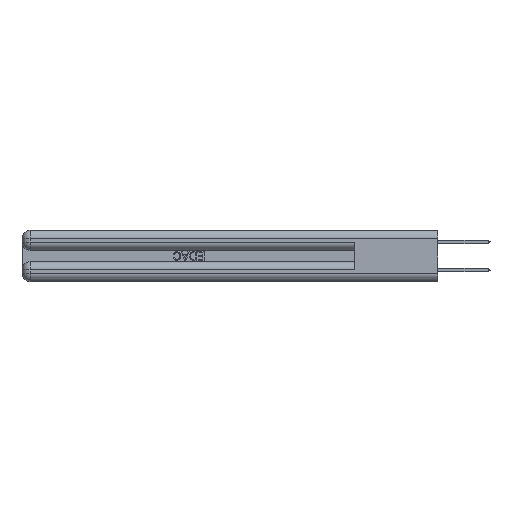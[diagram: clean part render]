
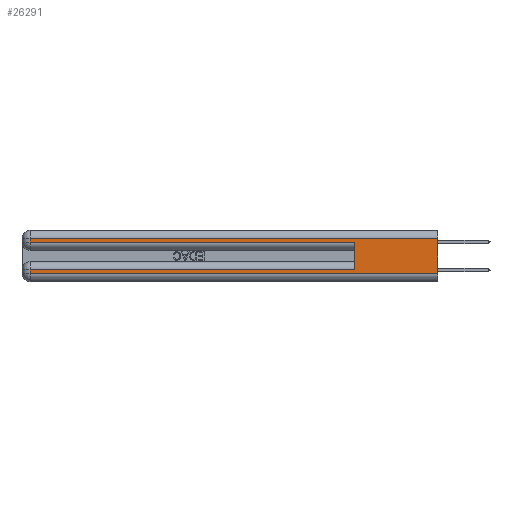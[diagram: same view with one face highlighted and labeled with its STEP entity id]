
A CAD part, left-side view. The second image highlights one B-rep face of the part: STEP entity #26291.
In plain terms, the highlighted planar face has unit normal (-1, 0, 0).
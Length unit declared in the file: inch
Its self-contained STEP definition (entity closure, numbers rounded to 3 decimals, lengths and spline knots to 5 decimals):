
#2 = LINE ( 'NONE', #25850, #28839 ) ;
#369 = VECTOR ( 'NONE', #11757, 39.37008 ) ;
#600 = CARTESIAN_POINT ( 'NONE',  ( 0., 0.6, 0.145 ) ) ;
#772 = VECTOR ( 'NONE', #30301, 39.37008 ) ;
#1163 = VERTEX_POINT ( 'NONE', #36578 ) ;
#1802 = VERTEX_POINT ( 'NONE', #23106 ) ;
#1910 = ORIENTED_EDGE ( 'NONE', *, *, #41942, .T. ) ;
#1934 = VERTEX_POINT ( 'NONE', #13478 ) ;
#3062 = CARTESIAN_POINT ( 'NONE',  ( 0., 2.94, 0.37 ) ) ;
#4387 = ORIENTED_EDGE ( 'NONE', *, *, #6411, .F. ) ;
#6411 = EDGE_CURVE ( 'NONE', #28365, #1802, #38617, .T. ) ;
#6689 = DIRECTION ( 'NONE',  ( 0., 0., -1. ) ) ;
#7509 = CARTESIAN_POINT ( 'NONE',  ( 0., 0., 0.285 ) ) ;
#8891 = CARTESIAN_POINT ( 'NONE',  ( 0., 2.94, 0.31 ) ) ;
#9011 = LINE ( 'NONE', #25058, #9567 ) ;
#9567 = VECTOR ( 'NONE', #35332, 39.37008 ) ;
#9829 = VERTEX_POINT ( 'NONE', #22189 ) ;
#9952 = EDGE_CURVE ( 'NONE', #9829, #1163, #9011, .T. ) ;
#9996 = DIRECTION ( 'NONE',  ( 0., -1., 0. ) ) ;
#11056 = CARTESIAN_POINT ( 'NONE',  ( 0., 0.6, 0.085 ) ) ;
#11757 = DIRECTION ( 'NONE',  ( 0., 0., -1. ) ) ;
#12996 = ORIENTED_EDGE ( 'NONE', *, *, #14078, .T. ) ;
#13316 = AXIS2_PLACEMENT_3D ( 'NONE', #23439, #39972, #6689 ) ;
#13478 = CARTESIAN_POINT ( 'NONE',  ( 0., 2.94, 0.285 ) ) ;
#13574 = DIRECTION ( 'NONE',  ( 0., 0., -1. ) ) ;
#13687 = VECTOR ( 'NONE', #9996, 39.37008 ) ;
#14078 = EDGE_CURVE ( 'NONE', #22019, #1163, #42571, .T. ) ;
#14930 = ORIENTED_EDGE ( 'NONE', *, *, #9952, .F. ) ;
#15753 = ORIENTED_EDGE ( 'NONE', *, *, #27311, .T. ) ;
#16132 = VECTOR ( 'NONE', #34354, 39.37008 ) ;
#17085 = EDGE_CURVE ( 'NONE', #28787, #22019, #27683, .T. ) ;
#17347 = LINE ( 'NONE', #3062, #39351 ) ;
#20038 = PLANE ( 'NONE',  #13316 ) ;
#20421 = ORIENTED_EDGE ( 'NONE', *, *, #34369, .T. ) ;
#21148 = CARTESIAN_POINT ( 'NONE',  ( 0., 2.94, 0.37 ) ) ;
#21474 = DIRECTION ( 'NONE',  ( 0., 1., 0. ) ) ;
#21560 = LINE ( 'NONE', #24256, #30461 ) ;
#22019 = VERTEX_POINT ( 'NONE', #38361 ) ;
#22189 = CARTESIAN_POINT ( 'NONE',  ( 0., 0., 0.31 ) ) ;
#22671 = CARTESIAN_POINT ( 'NONE',  ( 0., 2.94, 0.085 ) ) ;
#23106 = CARTESIAN_POINT ( 'NONE',  ( 0., 0.6, 0.285 ) ) ;
#23439 = CARTESIAN_POINT ( 'NONE',  ( 0., 0., 0.37 ) ) ;
#24256 = CARTESIAN_POINT ( 'NONE',  ( 0., 0., 0.085 ) ) ;
#25058 = CARTESIAN_POINT ( 'NONE',  ( 0., 0., 0.37 ) ) ;
#25850 = CARTESIAN_POINT ( 'NONE',  ( 0., 0., 0.31 ) ) ;
#26291 = ADVANCED_FACE ( 'NONE', ( #32659 ), #20038, .F. ) ;
#26771 = EDGE_LOOP ( 'NONE', ( #14930, #15753, #35998, #1910, #4387, #20421, #32830, #12996 ) ) ;
#27311 = EDGE_CURVE ( 'NONE', #9829, #42924, #2, .T. ) ;
#27683 = LINE ( 'NONE', #21148, #369 ) ;
#28224 = EDGE_CURVE ( 'NONE', #42924, #1934, #17347, .T. ) ;
#28365 = VERTEX_POINT ( 'NONE', #11056 ) ;
#28787 = VERTEX_POINT ( 'NONE', #22671 ) ;
#28839 = VECTOR ( 'NONE', #32600, 39.37008 ) ;
#30301 = DIRECTION ( 'NONE',  ( 0., 0., 1. ) ) ;
#30461 = VECTOR ( 'NONE', #21474, 39.37008 ) ;
#32439 = LINE ( 'NONE', #7509, #16132 ) ;
#32600 = DIRECTION ( 'NONE',  ( 0., 1., 0. ) ) ;
#32659 = FACE_OUTER_BOUND ( 'NONE', #26771, .T. ) ;
#32830 = ORIENTED_EDGE ( 'NONE', *, *, #17085, .T. ) ;
#34354 = DIRECTION ( 'NONE',  ( 0., -1., 0. ) ) ;
#34369 = EDGE_CURVE ( 'NONE', #28365, #28787, #21560, .T. ) ;
#35332 = DIRECTION ( 'NONE',  ( 0., 0., -1. ) ) ;
#35998 = ORIENTED_EDGE ( 'NONE', *, *, #28224, .T. ) ;
#36390 = CARTESIAN_POINT ( 'NONE',  ( 0., 0., 0.06 ) ) ;
#36578 = CARTESIAN_POINT ( 'NONE',  ( 0., 0., 0.06 ) ) ;
#38361 = CARTESIAN_POINT ( 'NONE',  ( 0., 2.94, 0.06 ) ) ;
#38617 = LINE ( 'NONE', #600, #772 ) ;
#39351 = VECTOR ( 'NONE', #13574, 39.37008 ) ;
#39972 = DIRECTION ( 'NONE',  ( 1., 0., 0. ) ) ;
#41942 = EDGE_CURVE ( 'NONE', #1934, #1802, #32439, .T. ) ;
#42571 = LINE ( 'NONE', #36390, #13687 ) ;
#42924 = VERTEX_POINT ( 'NONE', #8891 ) ;
